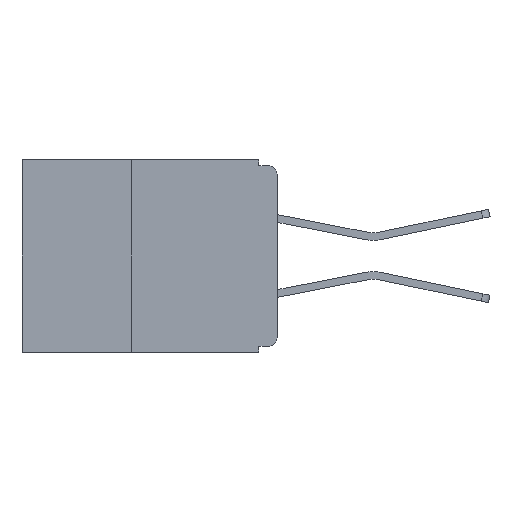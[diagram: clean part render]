
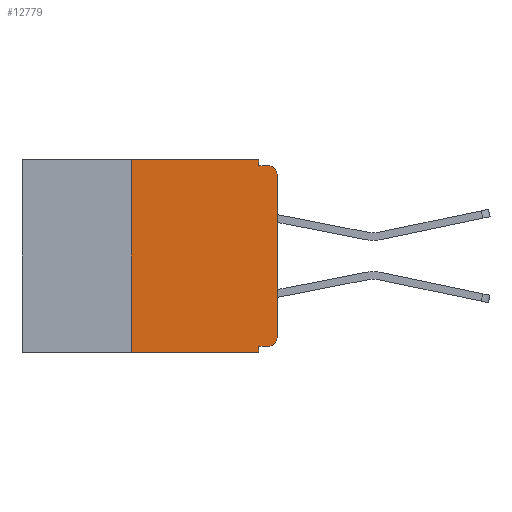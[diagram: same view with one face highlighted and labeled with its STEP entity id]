
A CAD part, left-side view. The second image highlights one B-rep face of the part: STEP entity #12779.
In plain terms, the highlighted planar face has unit normal (-1, 0, 0).
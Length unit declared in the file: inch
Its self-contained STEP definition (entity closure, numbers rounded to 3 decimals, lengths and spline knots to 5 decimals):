
#271 = VERTEX_POINT ( 'NONE', #27669 ) ;
#487 = DIRECTION ( 'NONE',  ( 1., 0., 0. ) ) ;
#750 = CARTESIAN_POINT ( 'NONE',  ( 0., 0.25, 0. ) ) ;
#2396 = AXIS2_PLACEMENT_3D ( 'NONE', #24701, #11687, #26854 ) ;
#2844 = DIRECTION ( 'NONE',  ( 0., 0., 1. ) ) ;
#3252 = EDGE_CURVE ( 'NONE', #15465, #21697, #16307, .T. ) ;
#3507 = VECTOR ( 'NONE', #22014, 39.37008 ) ;
#4029 = LINE ( 'NONE', #4440, #25890 ) ;
#4297 = CARTESIAN_POINT ( 'NONE',  ( 0., 0., 0. ) ) ;
#4440 = CARTESIAN_POINT ( 'NONE',  ( 0., 0.437, -0.33 ) ) ;
#4900 = VECTOR ( 'NONE', #10382, 39.37008 ) ;
#5402 = VERTEX_POINT ( 'NONE', #19353 ) ;
#5773 = CARTESIAN_POINT ( 'NONE',  ( 0., 0., -0.32 ) ) ;
#5984 = ORIENTED_EDGE ( 'NONE', *, *, #20091, .F. ) ;
#6225 = DIRECTION ( 'NONE',  ( 0., 0., -1. ) ) ;
#6861 = EDGE_LOOP ( 'NONE', ( #22976, #12133, #25052, #8392, #26391, #5984, #17561, #18906, #24724, #14514 ) ) ;
#7061 = VERTEX_POINT ( 'NONE', #16457 ) ;
#7500 = CARTESIAN_POINT ( 'NONE',  ( 0., 0.031, 0. ) ) ;
#7602 = DIRECTION ( 'NONE',  ( -1., 0., 0. ) ) ;
#8392 = ORIENTED_EDGE ( 'NONE', *, *, #21585, .F. ) ;
#8449 = VECTOR ( 'NONE', #6225, 39.37008 ) ;
#9237 = EDGE_CURVE ( 'NONE', #271, #5402, #28406, .T. ) ;
#9522 = CARTESIAN_POINT ( 'NONE',  ( 0., 0.015, -0.32 ) ) ;
#9683 = EDGE_CURVE ( 'NONE', #16832, #25043, #12860, .T. ) ;
#10382 = DIRECTION ( 'NONE',  ( 0., -1., 0. ) ) ;
#10754 = EDGE_CURVE ( 'NONE', #7061, #5402, #28024, .T. ) ;
#11544 = VECTOR ( 'NONE', #2844, 39.37008 ) ;
#11665 = CARTESIAN_POINT ( 'NONE',  ( 0., 0.437, 0. ) ) ;
#11687 = DIRECTION ( 'NONE',  ( -1., 0., 0. ) ) ;
#12133 = ORIENTED_EDGE ( 'NONE', *, *, #9237, .T. ) ;
#12378 = CARTESIAN_POINT ( 'NONE',  ( 0., 0.031, -0.33 ) ) ;
#12779 = ADVANCED_FACE ( 'NONE', ( #23920 ), #13846, .F. ) ;
#12860 = LINE ( 'NONE', #15271, #23736 ) ;
#13261 = CARTESIAN_POINT ( 'NONE',  ( 0., 0.031, 0. ) ) ;
#13846 = PLANE ( 'NONE',  #19783 ) ;
#14229 = LINE ( 'NONE', #19229, #8449 ) ;
#14514 = ORIENTED_EDGE ( 'NONE', *, *, #3252, .T. ) ;
#14887 = VECTOR ( 'NONE', #19548, 39.37008 ) ;
#15197 = LINE ( 'NONE', #13261, #3507 ) ;
#15271 = CARTESIAN_POINT ( 'NONE',  ( 0., 0.437, 0. ) ) ;
#15465 = VERTEX_POINT ( 'NONE', #9522 ) ;
#15765 = EDGE_CURVE ( 'NONE', #18450, #24566, #14229, .T. ) ;
#16020 = DIRECTION ( 'NONE',  ( 0., 0., -1. ) ) ;
#16307 = CIRCLE ( 'NONE', #28438, 0.015 ) ;
#16457 = CARTESIAN_POINT ( 'NONE',  ( 0., 0.031, -0.01 ) ) ;
#16832 = VERTEX_POINT ( 'NONE', #750 ) ;
#16864 = CARTESIAN_POINT ( 'NONE',  ( 0., 0.031, -0.32 ) ) ;
#16901 = CARTESIAN_POINT ( 'NONE',  ( 0., 0., -0.01 ) ) ;
#17293 = LINE ( 'NONE', #22486, #11544 ) ;
#17433 = DIRECTION ( 'NONE',  ( 0., -1., 0. ) ) ;
#17561 = ORIENTED_EDGE ( 'NONE', *, *, #18634, .T. ) ;
#18450 = VERTEX_POINT ( 'NONE', #16864 ) ;
#18634 = EDGE_CURVE ( 'NONE', #27072, #24566, #4029, .T. ) ;
#18906 = ORIENTED_EDGE ( 'NONE', *, *, #15765, .F. ) ;
#19229 = CARTESIAN_POINT ( 'NONE',  ( 0., 0.031, -0.33 ) ) ;
#19353 = CARTESIAN_POINT ( 'NONE',  ( 0., 0.015, -0.01 ) ) ;
#19548 = DIRECTION ( 'NONE',  ( 0., 0., 1. ) ) ;
#19783 = AXIS2_PLACEMENT_3D ( 'NONE', #11665, #487, #16020 ) ;
#20091 = EDGE_CURVE ( 'NONE', #27072, #16832, #17293, .T. ) ;
#20161 = CARTESIAN_POINT ( 'NONE',  ( 0., 0., -0.305 ) ) ;
#20301 = LINE ( 'NONE', #5773, #25433 ) ;
#20601 = CARTESIAN_POINT ( 'NONE',  ( 0., 0.015, -0.305 ) ) ;
#20692 = EDGE_CURVE ( 'NONE', #15465, #18450, #20301, .T. ) ;
#20910 = EDGE_CURVE ( 'NONE', #21697, #271, #26432, .T. ) ;
#21433 = CARTESIAN_POINT ( 'NONE',  ( 0., 0.25, -0.33 ) ) ;
#21585 = EDGE_CURVE ( 'NONE', #25043, #7061, #15197, .T. ) ;
#21697 = VERTEX_POINT ( 'NONE', #20161 ) ;
#22014 = DIRECTION ( 'NONE',  ( 0., 0., -1. ) ) ;
#22486 = CARTESIAN_POINT ( 'NONE',  ( 0., 0.25, -0.33 ) ) ;
#22800 = DIRECTION ( 'NONE',  ( 0., 0., -1. ) ) ;
#22976 = ORIENTED_EDGE ( 'NONE', *, *, #20910, .T. ) ;
#23185 = DIRECTION ( 'NONE',  ( 0., 1., 0. ) ) ;
#23736 = VECTOR ( 'NONE', #17433, 39.37008 ) ;
#23920 = FACE_OUTER_BOUND ( 'NONE', #6861, .T. ) ;
#24566 = VERTEX_POINT ( 'NONE', #12378 ) ;
#24701 = CARTESIAN_POINT ( 'NONE',  ( 0., 0.015, -0.025 ) ) ;
#24724 = ORIENTED_EDGE ( 'NONE', *, *, #20692, .F. ) ;
#25043 = VERTEX_POINT ( 'NONE', #7500 ) ;
#25052 = ORIENTED_EDGE ( 'NONE', *, *, #10754, .F. ) ;
#25433 = VECTOR ( 'NONE', #23185, 39.37008 ) ;
#25890 = VECTOR ( 'NONE', #28286, 39.37008 ) ;
#26391 = ORIENTED_EDGE ( 'NONE', *, *, #9683, .F. ) ;
#26432 = LINE ( 'NONE', #4297, #14887 ) ;
#26854 = DIRECTION ( 'NONE',  ( 0., 0., -1. ) ) ;
#27072 = VERTEX_POINT ( 'NONE', #21433 ) ;
#27669 = CARTESIAN_POINT ( 'NONE',  ( 0., 0., -0.025 ) ) ;
#28024 = LINE ( 'NONE', #16901, #4900 ) ;
#28286 = DIRECTION ( 'NONE',  ( 0., -1., 0. ) ) ;
#28406 = CIRCLE ( 'NONE', #2396, 0.015 ) ;
#28438 = AXIS2_PLACEMENT_3D ( 'NONE', #20601, #7602, #22800 ) ;
